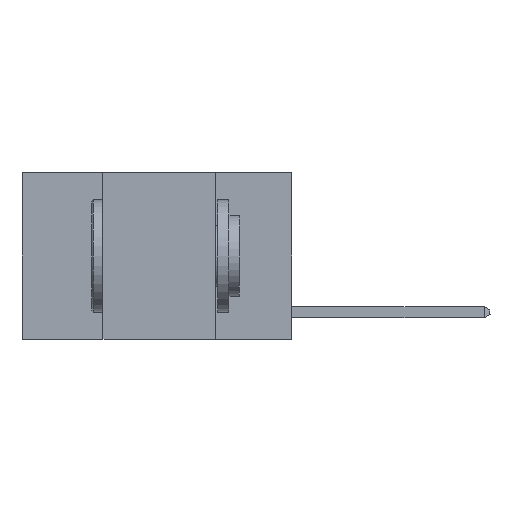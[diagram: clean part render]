
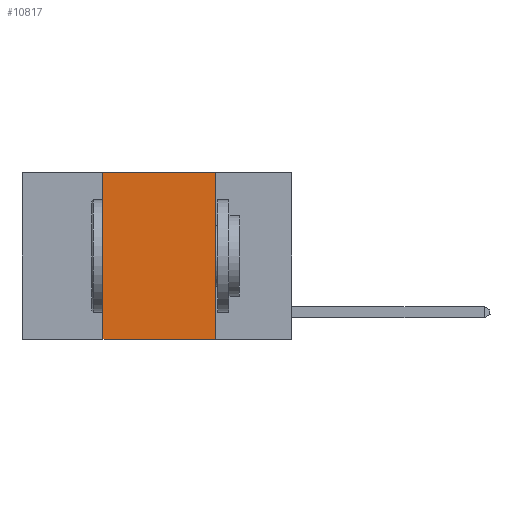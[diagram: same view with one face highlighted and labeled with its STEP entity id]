
A CAD part, left-side view. The second image highlights one B-rep face of the part: STEP entity #10817.
In plain terms, the highlighted planar face has unit normal (-1, 0, 0).
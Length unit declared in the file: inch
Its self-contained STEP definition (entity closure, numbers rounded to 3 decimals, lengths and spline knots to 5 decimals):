
#63 = EDGE_CURVE ( 'NONE', #665, #11133, #2458, .T. ) ;
#297 = EDGE_LOOP ( 'NONE', ( #1617, #9719, #10971, #3352 ) ) ;
#665 = VERTEX_POINT ( 'NONE', #6150 ) ;
#702 = EDGE_CURVE ( 'NONE', #7887, #665, #4811, .T. ) ;
#1617 = ORIENTED_EDGE ( 'NONE', *, *, #63, .F. ) ;
#2224 = EDGE_CURVE ( 'NONE', #2723, #7887, #7429, .T. ) ;
#2349 = CARTESIAN_POINT ( 'NONE',  ( 0., 0.42, -0.37 ) ) ;
#2355 = CARTESIAN_POINT ( 'NONE',  ( 0., 0.6, 0. ) ) ;
#2458 = LINE ( 'NONE', #10345, #9905 ) ;
#2723 = VERTEX_POINT ( 'NONE', #2349 ) ;
#3352 = ORIENTED_EDGE ( 'NONE', *, *, #12232, .T. ) ;
#3359 = PLANE ( 'NONE',  #11297 ) ;
#4341 = DIRECTION ( 'NONE',  ( 0., 0., 1. ) ) ;
#4773 = LINE ( 'NONE', #8714, #7253 ) ;
#4811 = LINE ( 'NONE', #11938, #8586 ) ;
#5211 = CARTESIAN_POINT ( 'NONE',  ( 0., 0.17, -0.37 ) ) ;
#6150 = CARTESIAN_POINT ( 'NONE',  ( 0., 0.17, 0. ) ) ;
#6574 = DIRECTION ( 'NONE',  ( 0., 0., -1. ) ) ;
#6990 = CARTESIAN_POINT ( 'NONE',  ( 0., 0.42, 0. ) ) ;
#7253 = VECTOR ( 'NONE', #10780, 39.37008 ) ;
#7267 = FACE_OUTER_BOUND ( 'NONE', #297, .T. ) ;
#7429 = LINE ( 'NONE', #9473, #9788 ) ;
#7887 = VERTEX_POINT ( 'NONE', #6990 ) ;
#8455 = DIRECTION ( 'NONE',  ( 0., 0., -1. ) ) ;
#8586 = VECTOR ( 'NONE', #10272, 39.37008 ) ;
#8714 = CARTESIAN_POINT ( 'NONE',  ( 0., 0.6, -0.37 ) ) ;
#9473 = CARTESIAN_POINT ( 'NONE',  ( 0., 0.42, 0. ) ) ;
#9719 = ORIENTED_EDGE ( 'NONE', *, *, #702, .F. ) ;
#9788 = VECTOR ( 'NONE', #4341, 39.37008 ) ;
#9905 = VECTOR ( 'NONE', #6574, 39.37008 ) ;
#10272 = DIRECTION ( 'NONE',  ( 0., -1., 0. ) ) ;
#10345 = CARTESIAN_POINT ( 'NONE',  ( 0., 0.17, 0. ) ) ;
#10780 = DIRECTION ( 'NONE',  ( 0., -1., 0. ) ) ;
#10817 = ADVANCED_FACE ( 'NONE', ( #7267 ), #3359, .F. ) ;
#10971 = ORIENTED_EDGE ( 'NONE', *, *, #2224, .F. ) ;
#11133 = VERTEX_POINT ( 'NONE', #5211 ) ;
#11297 = AXIS2_PLACEMENT_3D ( 'NONE', #2355, #11326, #8455 ) ;
#11326 = DIRECTION ( 'NONE',  ( 1., 0., 0. ) ) ;
#11938 = CARTESIAN_POINT ( 'NONE',  ( 0., 0.6, 0. ) ) ;
#12232 = EDGE_CURVE ( 'NONE', #2723, #11133, #4773, .T. ) ;
